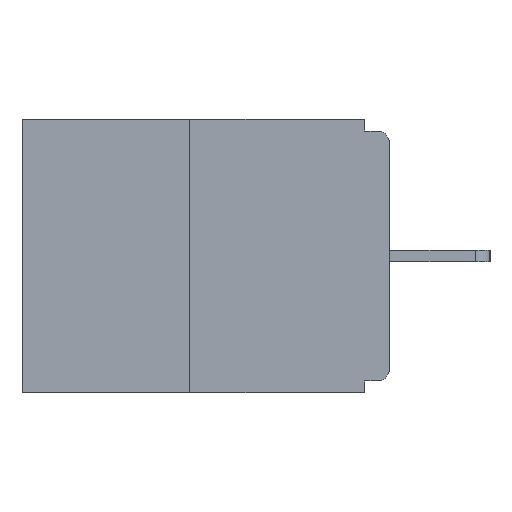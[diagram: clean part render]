
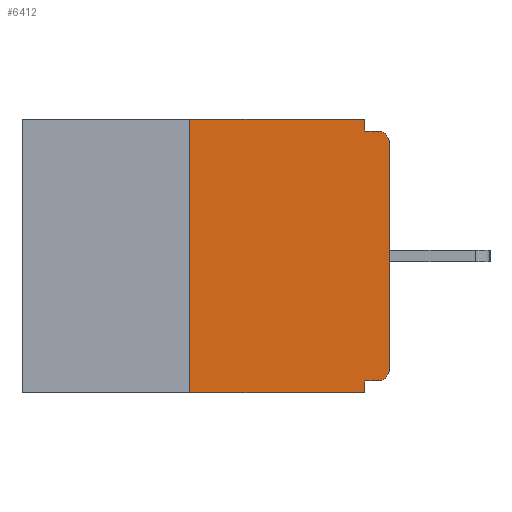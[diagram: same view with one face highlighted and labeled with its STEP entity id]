
A CAD part, left-side view. The second image highlights one B-rep face of the part: STEP entity #6412.
In plain terms, the highlighted planar face has unit normal (-1, 0, 0).
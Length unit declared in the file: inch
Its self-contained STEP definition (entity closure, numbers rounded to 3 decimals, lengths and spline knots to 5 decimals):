
#211 = VERTEX_POINT ( 'NONE', #16547 ) ;
#500 = EDGE_CURVE ( 'NONE', #1441, #15984, #2628, .T. ) ;
#764 = VERTEX_POINT ( 'NONE', #10389 ) ;
#788 = CARTESIAN_POINT ( 'NONE',  ( 0., 0.25, -0.343 ) ) ;
#1129 = ORIENTED_EDGE ( 'NONE', *, *, #7538, .F. ) ;
#1146 = DIRECTION ( 'NONE',  ( 0., 1., 0. ) ) ;
#1441 = VERTEX_POINT ( 'NONE', #16053 ) ;
#1453 = CARTESIAN_POINT ( 'NONE',  ( 0., 0.031, 0. ) ) ;
#1456 = EDGE_CURVE ( 'NONE', #2442, #211, #13163, .T. ) ;
#1736 = CARTESIAN_POINT ( 'NONE',  ( 0., 0.031, -0.343 ) ) ;
#1741 = CARTESIAN_POINT ( 'NONE',  ( 0., 0.46, 0. ) ) ;
#2245 = CARTESIAN_POINT ( 'NONE',  ( 0., 0.25, 0. ) ) ;
#2308 = CIRCLE ( 'NONE', #12714, 0.015 ) ;
#2442 = VERTEX_POINT ( 'NONE', #9824 ) ;
#2628 = LINE ( 'NONE', #1453, #9826 ) ;
#2880 = VERTEX_POINT ( 'NONE', #3154 ) ;
#3154 = CARTESIAN_POINT ( 'NONE',  ( 0., 0., -0.313 ) ) ;
#3562 = PLANE ( 'NONE',  #17164 ) ;
#3622 = DIRECTION ( 'NONE',  ( -1., 0., 0. ) ) ;
#3973 = EDGE_CURVE ( 'NONE', #8665, #9722, #17125, .T. ) ;
#4060 = CARTESIAN_POINT ( 'NONE',  ( 0., 0., -0.03 ) ) ;
#4264 = VECTOR ( 'NONE', #15036, 39.37008 ) ;
#4712 = VERTEX_POINT ( 'NONE', #788 ) ;
#4916 = FACE_OUTER_BOUND ( 'NONE', #13594, .T. ) ;
#5098 = DIRECTION ( 'NONE',  ( 0., 0., 1. ) ) ;
#5511 = VECTOR ( 'NONE', #1146, 39.37008 ) ;
#5694 = CARTESIAN_POINT ( 'NONE',  ( 0., 0.46, -0.343 ) ) ;
#5909 = LINE ( 'NONE', #1741, #17318 ) ;
#5958 = LINE ( 'NONE', #9702, #4264 ) ;
#6068 = CARTESIAN_POINT ( 'NONE',  ( 0., 0.25, 0. ) ) ;
#6262 = CARTESIAN_POINT ( 'NONE',  ( 0., 0.015, -0.015 ) ) ;
#6386 = DIRECTION ( 'NONE',  ( 0., 0., -1. ) ) ;
#6412 = ADVANCED_FACE ( 'NONE', ( #4916 ), #3562, .F. ) ;
#6885 = ORIENTED_EDGE ( 'NONE', *, *, #10505, .T. ) ;
#7014 = ORIENTED_EDGE ( 'NONE', *, *, #13551, .F. ) ;
#7276 = LINE ( 'NONE', #5694, #17257 ) ;
#7401 = LINE ( 'NONE', #6068, #10595 ) ;
#7538 = EDGE_CURVE ( 'NONE', #15984, #9722, #5958, .T. ) ;
#7575 = DIRECTION ( 'NONE',  ( 0., 0., -1. ) ) ;
#7608 = VERTEX_POINT ( 'NONE', #2245 ) ;
#8097 = ORIENTED_EDGE ( 'NONE', *, *, #15952, .T. ) ;
#8562 = DIRECTION ( 'NONE',  ( 0., 0., -1. ) ) ;
#8630 = VECTOR ( 'NONE', #5098, 39.37008 ) ;
#8665 = VERTEX_POINT ( 'NONE', #4060 ) ;
#8799 = DIRECTION ( 'NONE',  ( 1., 0., 0. ) ) ;
#8943 = CARTESIAN_POINT ( 'NONE',  ( 0., 0.015, -0.03 ) ) ;
#9025 = DIRECTION ( 'NONE',  ( 0., 0., -1. ) ) ;
#9702 = CARTESIAN_POINT ( 'NONE',  ( 0., 0., -0.015 ) ) ;
#9722 = VERTEX_POINT ( 'NONE', #6262 ) ;
#9802 = ORIENTED_EDGE ( 'NONE', *, *, #1456, .F. ) ;
#9824 = CARTESIAN_POINT ( 'NONE',  ( 0., 0.015, -0.328 ) ) ;
#9826 = VECTOR ( 'NONE', #13645, 39.37008 ) ;
#10070 = EDGE_CURVE ( 'NONE', #211, #764, #13580, .T. ) ;
#10389 = CARTESIAN_POINT ( 'NONE',  ( 0., 0.031, -0.343 ) ) ;
#10505 = EDGE_CURVE ( 'NONE', #2442, #2880, #2308, .T. ) ;
#10561 = CARTESIAN_POINT ( 'NONE',  ( 0., 0.031, -0.015 ) ) ;
#10595 = VECTOR ( 'NONE', #10665, 39.37008 ) ;
#10665 = DIRECTION ( 'NONE',  ( 0., 0., 1. ) ) ;
#10767 = VECTOR ( 'NONE', #8562, 39.37008 ) ;
#11076 = DIRECTION ( 'NONE',  ( 0., -1., 0. ) ) ;
#11228 = AXIS2_PLACEMENT_3D ( 'NONE', #8943, #3622, #9025 ) ;
#11287 = DIRECTION ( 'NONE',  ( 0., -1., 0. ) ) ;
#11392 = ORIENTED_EDGE ( 'NONE', *, *, #13447, .F. ) ;
#11393 = EDGE_CURVE ( 'NONE', #4712, #764, #7276, .T. ) ;
#11525 = ORIENTED_EDGE ( 'NONE', *, *, #11393, .T. ) ;
#11532 = DIRECTION ( 'NONE',  ( -1., 0., 0. ) ) ;
#11684 = CARTESIAN_POINT ( 'NONE',  ( 0., 0.46, 0. ) ) ;
#11778 = LINE ( 'NONE', #15450, #8630 ) ;
#12714 = AXIS2_PLACEMENT_3D ( 'NONE', #14013, #11532, #7575 ) ;
#13163 = LINE ( 'NONE', #15875, #5511 ) ;
#13447 = EDGE_CURVE ( 'NONE', #7608, #1441, #5909, .T. ) ;
#13551 = EDGE_CURVE ( 'NONE', #4712, #7608, #7401, .T. ) ;
#13580 = LINE ( 'NONE', #1736, #10767 ) ;
#13594 = EDGE_LOOP ( 'NONE', ( #11392, #7014, #11525, #15596, #9802, #6885, #8097, #14857, #1129, #14107 ) ) ;
#13645 = DIRECTION ( 'NONE',  ( 0., 0., -1. ) ) ;
#14013 = CARTESIAN_POINT ( 'NONE',  ( 0., 0.015, -0.313 ) ) ;
#14107 = ORIENTED_EDGE ( 'NONE', *, *, #500, .F. ) ;
#14857 = ORIENTED_EDGE ( 'NONE', *, *, #3973, .T. ) ;
#15036 = DIRECTION ( 'NONE',  ( 0., -1., 0. ) ) ;
#15450 = CARTESIAN_POINT ( 'NONE',  ( 0., 0., 0. ) ) ;
#15596 = ORIENTED_EDGE ( 'NONE', *, *, #10070, .F. ) ;
#15875 = CARTESIAN_POINT ( 'NONE',  ( 0., 0., -0.328 ) ) ;
#15952 = EDGE_CURVE ( 'NONE', #2880, #8665, #11778, .T. ) ;
#15984 = VERTEX_POINT ( 'NONE', #10561 ) ;
#16053 = CARTESIAN_POINT ( 'NONE',  ( 0., 0.031, 0. ) ) ;
#16547 = CARTESIAN_POINT ( 'NONE',  ( 0., 0.031, -0.328 ) ) ;
#17125 = CIRCLE ( 'NONE', #11228, 0.015 ) ;
#17164 = AXIS2_PLACEMENT_3D ( 'NONE', #11684, #8799, #6386 ) ;
#17257 = VECTOR ( 'NONE', #11076, 39.37008 ) ;
#17318 = VECTOR ( 'NONE', #11287, 39.37008 ) ;
